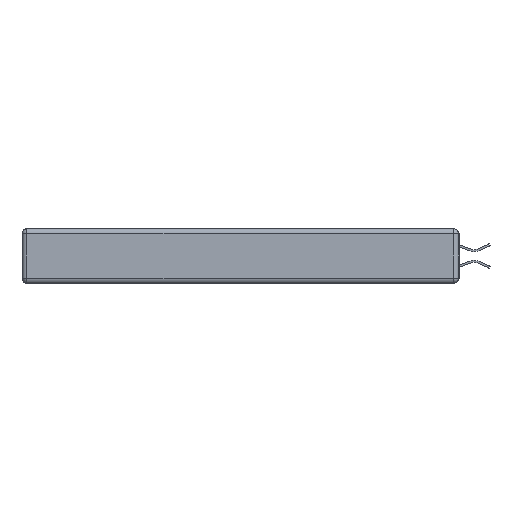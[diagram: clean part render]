
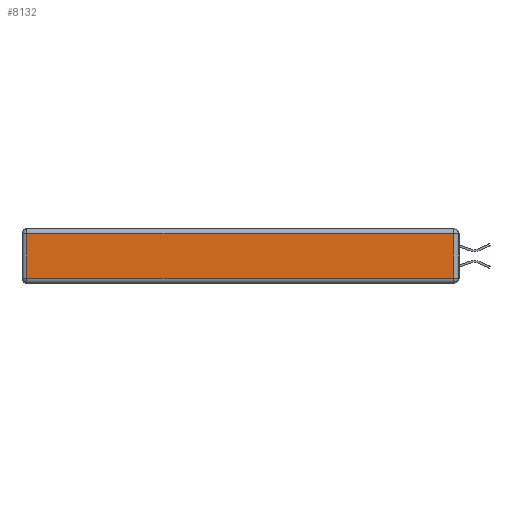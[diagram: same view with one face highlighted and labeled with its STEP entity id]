
A CAD part, left-side view. The second image highlights one B-rep face of the part: STEP entity #8132.
In plain terms, the highlighted planar face has unit normal (-1, 0, 0).
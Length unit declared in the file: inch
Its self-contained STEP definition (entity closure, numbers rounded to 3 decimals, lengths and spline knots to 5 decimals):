
#485 = EDGE_CURVE ( 'NONE', #12819, #6942, #22258, .T. ) ;
#1033 = LINE ( 'NONE', #13084, #4596 ) ;
#1038 = VECTOR ( 'NONE', #2783, 39.37008 ) ;
#1332 = EDGE_CURVE ( 'NONE', #10992, #11235, #17067, .T. ) ;
#2783 = DIRECTION ( 'NONE',  ( 0., -1., 0. ) ) ;
#3697 = AXIS2_PLACEMENT_3D ( 'NONE', #8349, #6461, #11730 ) ;
#4143 = ORIENTED_EDGE ( 'NONE', *, *, #11106, .T. ) ;
#4292 = FACE_OUTER_BOUND ( 'NONE', #18749, .T. ) ;
#4596 = VECTOR ( 'NONE', #16557, 39.37008 ) ;
#4658 = DIRECTION ( 'NONE',  ( 0., 0., 1. ) ) ;
#4959 = PLANE ( 'NONE',  #3697 ) ;
#6461 = DIRECTION ( 'NONE',  ( -1., 0., 0. ) ) ;
#6942 = VERTEX_POINT ( 'NONE', #9897 ) ;
#7937 = CARTESIAN_POINT ( 'NONE',  ( 0., 2.75, -0.03 ) ) ;
#8132 = ADVANCED_FACE ( 'NONE', ( #4292 ), #4959, .T. ) ;
#8349 = CARTESIAN_POINT ( 'NONE',  ( 0., 0., -0.343 ) ) ;
#9013 = CARTESIAN_POINT ( 'NONE',  ( 0., 0.03, -0.03 ) ) ;
#9677 = DIRECTION ( 'NONE',  ( 0., 1., 0. ) ) ;
#9897 = CARTESIAN_POINT ( 'NONE',  ( 0., 0.03, -0.313 ) ) ;
#10992 = VERTEX_POINT ( 'NONE', #9013 ) ;
#11106 = EDGE_CURVE ( 'NONE', #6942, #10992, #13402, .T. ) ;
#11235 = VERTEX_POINT ( 'NONE', #11901 ) ;
#11569 = ORIENTED_EDGE ( 'NONE', *, *, #485, .T. ) ;
#11730 = DIRECTION ( 'NONE',  ( 0., 0., 1. ) ) ;
#11901 = CARTESIAN_POINT ( 'NONE',  ( 0., 2.72, -0.03 ) ) ;
#12819 = VERTEX_POINT ( 'NONE', #22182 ) ;
#13084 = CARTESIAN_POINT ( 'NONE',  ( 0., 2.72, -0.343 ) ) ;
#13402 = LINE ( 'NONE', #15074, #14201 ) ;
#14201 = VECTOR ( 'NONE', #4658, 39.37008 ) ;
#14732 = CARTESIAN_POINT ( 'NONE',  ( 0., 0., -0.313 ) ) ;
#14794 = ORIENTED_EDGE ( 'NONE', *, *, #1332, .T. ) ;
#15074 = CARTESIAN_POINT ( 'NONE',  ( 0., 0.03, -0.343 ) ) ;
#15731 = VECTOR ( 'NONE', #9677, 39.37008 ) ;
#16557 = DIRECTION ( 'NONE',  ( 0., 0., -1. ) ) ;
#17067 = LINE ( 'NONE', #7937, #15731 ) ;
#18749 = EDGE_LOOP ( 'NONE', ( #11569, #4143, #14794, #21889 ) ) ;
#19105 = EDGE_CURVE ( 'NONE', #11235, #12819, #1033, .T. ) ;
#21889 = ORIENTED_EDGE ( 'NONE', *, *, #19105, .T. ) ;
#22182 = CARTESIAN_POINT ( 'NONE',  ( 0., 2.72, -0.313 ) ) ;
#22258 = LINE ( 'NONE', #14732, #1038 ) ;
